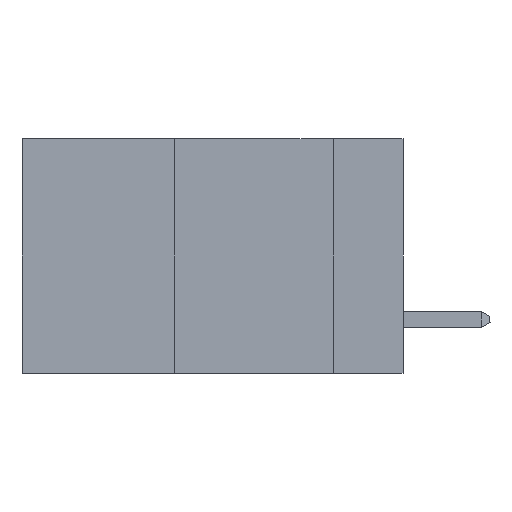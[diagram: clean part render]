
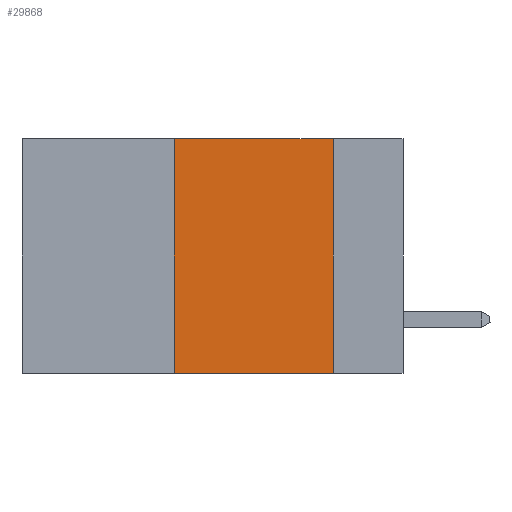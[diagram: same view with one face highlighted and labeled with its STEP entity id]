
A CAD part, left-side view. The second image highlights one B-rep face of the part: STEP entity #29868.
In plain terms, the highlighted planar face has unit normal (-1, 0, 0).
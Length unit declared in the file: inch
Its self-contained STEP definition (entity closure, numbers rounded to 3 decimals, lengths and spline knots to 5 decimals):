
#158 = VERTEX_POINT ( 'NONE', #37676 ) ;
#815 = CARTESIAN_POINT ( 'NONE',  ( 0., 0.6, -0.37 ) ) ;
#2057 = LINE ( 'NONE', #815, #39100 ) ;
#2407 = LINE ( 'NONE', #36526, #29385 ) ;
#6633 = ORIENTED_EDGE ( 'NONE', *, *, #21764, .F. ) ;
#7848 = ORIENTED_EDGE ( 'NONE', *, *, #13628, .T. ) ;
#7941 = PLANE ( 'NONE',  #10591 ) ;
#8165 = LINE ( 'NONE', #45296, #13016 ) ;
#10584 = VERTEX_POINT ( 'NONE', #24483 ) ;
#10591 = AXIS2_PLACEMENT_3D ( 'NONE', #36592, #33910, #30333 ) ;
#11437 = CARTESIAN_POINT ( 'NONE',  ( 0., 0.36, 0. ) ) ;
#12610 = EDGE_CURVE ( 'NONE', #17366, #158, #8165, .T. ) ;
#13016 = VECTOR ( 'NONE', #37579, 39.37008 ) ;
#13306 = CARTESIAN_POINT ( 'NONE',  ( 0., 0.36, 0. ) ) ;
#13628 = EDGE_CURVE ( 'NONE', #10584, #158, #2057, .T. ) ;
#15493 = EDGE_CURVE ( 'NONE', #44892, #17366, #2407, .T. ) ;
#17366 = VERTEX_POINT ( 'NONE', #20757 ) ;
#19152 = DIRECTION ( 'NONE',  ( 0., -1., 0. ) ) ;
#20757 = CARTESIAN_POINT ( 'NONE',  ( 0., 0.11, 0. ) ) ;
#21764 = EDGE_CURVE ( 'NONE', #10584, #44892, #44395, .T. ) ;
#22549 = DIRECTION ( 'NONE',  ( 0., -1., 0. ) ) ;
#23599 = ORIENTED_EDGE ( 'NONE', *, *, #15493, .F. ) ;
#24483 = CARTESIAN_POINT ( 'NONE',  ( 0., 0.36, -0.37 ) ) ;
#25224 = EDGE_LOOP ( 'NONE', ( #42779, #23599, #6633, #7848 ) ) ;
#29385 = VECTOR ( 'NONE', #19152, 39.37008 ) ;
#29868 = ADVANCED_FACE ( 'NONE', ( #35916 ), #7941, .F. ) ;
#30333 = DIRECTION ( 'NONE',  ( 0., 0., -1. ) ) ;
#33910 = DIRECTION ( 'NONE',  ( 1., 0., 0. ) ) ;
#35916 = FACE_OUTER_BOUND ( 'NONE', #25224, .T. ) ;
#36526 = CARTESIAN_POINT ( 'NONE',  ( 0., 0.6, 0. ) ) ;
#36592 = CARTESIAN_POINT ( 'NONE',  ( 0., 0.6, 0. ) ) ;
#37579 = DIRECTION ( 'NONE',  ( 0., 0., -1. ) ) ;
#37676 = CARTESIAN_POINT ( 'NONE',  ( 0., 0.11, -0.37 ) ) ;
#39100 = VECTOR ( 'NONE', #22549, 39.37008 ) ;
#42779 = ORIENTED_EDGE ( 'NONE', *, *, #12610, .F. ) ;
#43801 = VECTOR ( 'NONE', #45552, 39.37008 ) ;
#44395 = LINE ( 'NONE', #13306, #43801 ) ;
#44892 = VERTEX_POINT ( 'NONE', #11437 ) ;
#45296 = CARTESIAN_POINT ( 'NONE',  ( 0., 0.11, 0. ) ) ;
#45552 = DIRECTION ( 'NONE',  ( 0., 0., 1. ) ) ;
